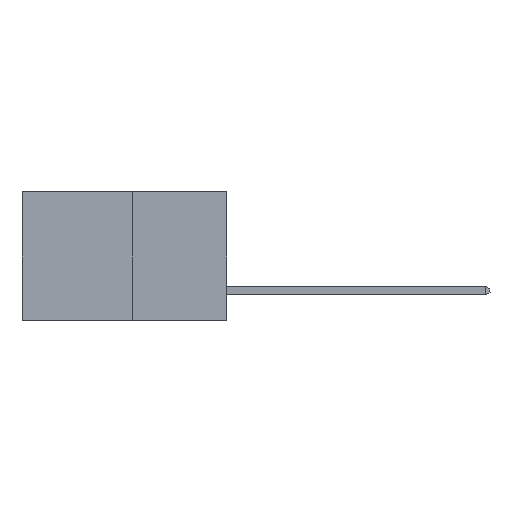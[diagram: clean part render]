
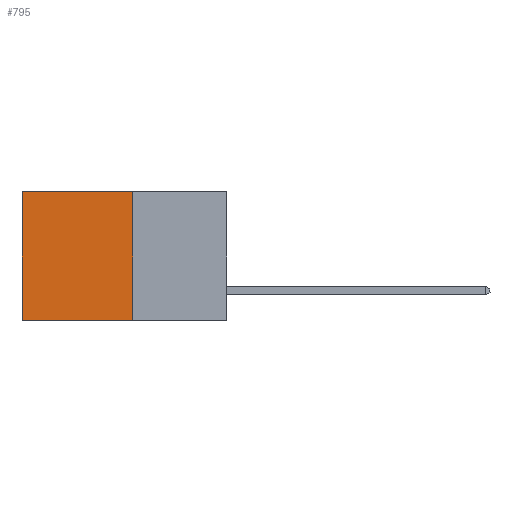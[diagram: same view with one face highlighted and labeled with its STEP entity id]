
A CAD part, left-side view. The second image highlights one B-rep face of the part: STEP entity #795.
In plain terms, the highlighted planar face has unit normal (-1, 0, 0).
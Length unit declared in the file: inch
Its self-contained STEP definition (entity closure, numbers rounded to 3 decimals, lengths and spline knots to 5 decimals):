
#41 = DIRECTION ( 'NONE',  ( 0., 1., 0. ) ) ;
#795 = ADVANCED_FACE ( 'NONE', ( #6028 ), #14852, .F. ) ;
#1463 = DIRECTION ( 'NONE',  ( 0., 0., -1. ) ) ;
#1482 = LINE ( 'NONE', #5033, #14011 ) ;
#2765 = LINE ( 'NONE', #11997, #14911 ) ;
#2818 = CARTESIAN_POINT ( 'NONE',  ( 0.277, 0.27, -0.37 ) ) ;
#3803 = ORIENTED_EDGE ( 'NONE', *, *, #4154, .F. ) ;
#3909 = VERTEX_POINT ( 'NONE', #5496 ) ;
#4154 = EDGE_CURVE ( 'NONE', #12734, #8078, #4424, .T. ) ;
#4424 = LINE ( 'NONE', #4703, #13754 ) ;
#4703 = CARTESIAN_POINT ( 'NONE',  ( 0.277, 0.27, -0.37 ) ) ;
#5033 = CARTESIAN_POINT ( 'NONE',  ( 0.277, 0.59, -0.37 ) ) ;
#5496 = CARTESIAN_POINT ( 'NONE',  ( 0.277, 0.59, -0.37 ) ) ;
#5651 = CARTESIAN_POINT ( 'NONE',  ( 0.277, 0.27, 0. ) ) ;
#6028 = FACE_OUTER_BOUND ( 'NONE', #13620, .T. ) ;
#7161 = EDGE_CURVE ( 'NONE', #12734, #13184, #2765, .T. ) ;
#8078 = VERTEX_POINT ( 'NONE', #2818 ) ;
#9705 = AXIS2_PLACEMENT_3D ( 'NONE', #14764, #11245, #11074 ) ;
#9954 = ORIENTED_EDGE ( 'NONE', *, *, #7161, .T. ) ;
#9974 = ORIENTED_EDGE ( 'NONE', *, *, #11885, .T. ) ;
#10042 = LINE ( 'NONE', #14554, #13302 ) ;
#10446 = EDGE_CURVE ( 'NONE', #8078, #3909, #10042, .T. ) ;
#11074 = DIRECTION ( 'NONE',  ( 0., 0., -1. ) ) ;
#11245 = DIRECTION ( 'NONE',  ( 1., 0., 0. ) ) ;
#11885 = EDGE_CURVE ( 'NONE', #13184, #3909, #1482, .T. ) ;
#11997 = CARTESIAN_POINT ( 'NONE',  ( 0.277, 0.27, 0. ) ) ;
#12029 = DIRECTION ( 'NONE',  ( 0., 0., -1. ) ) ;
#12613 = CARTESIAN_POINT ( 'NONE',  ( 0.277, 0.59, 0. ) ) ;
#12734 = VERTEX_POINT ( 'NONE', #5651 ) ;
#13184 = VERTEX_POINT ( 'NONE', #12613 ) ;
#13233 = DIRECTION ( 'NONE',  ( 0., 1., 0. ) ) ;
#13302 = VECTOR ( 'NONE', #41, 39.37008 ) ;
#13620 = EDGE_LOOP ( 'NONE', ( #9974, #15374, #3803, #9954 ) ) ;
#13754 = VECTOR ( 'NONE', #12029, 39.37008 ) ;
#14011 = VECTOR ( 'NONE', #1463, 39.37008 ) ;
#14554 = CARTESIAN_POINT ( 'NONE',  ( 0.277, 0.27, -0.37 ) ) ;
#14764 = CARTESIAN_POINT ( 'NONE',  ( 0.277, 0.27, -0.37 ) ) ;
#14852 = PLANE ( 'NONE',  #9705 ) ;
#14911 = VECTOR ( 'NONE', #13233, 39.37008 ) ;
#15374 = ORIENTED_EDGE ( 'NONE', *, *, #10446, .F. ) ;
